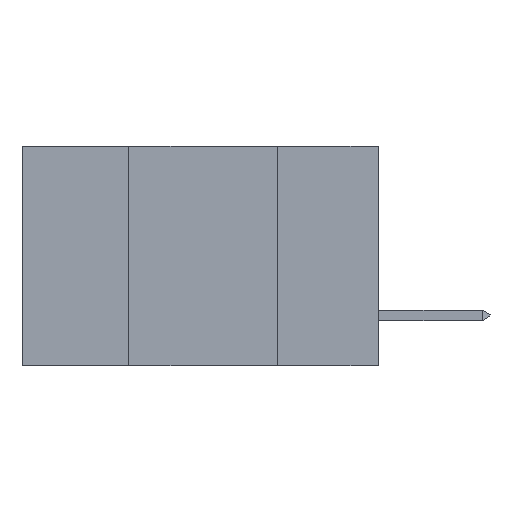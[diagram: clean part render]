
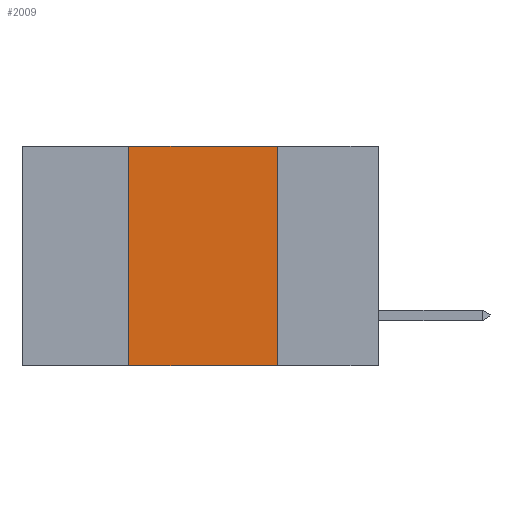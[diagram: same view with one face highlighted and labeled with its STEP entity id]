
A CAD part, left-side view. The second image highlights one B-rep face of the part: STEP entity #2009.
In plain terms, the highlighted planar face has unit normal (-1, 0, 0).
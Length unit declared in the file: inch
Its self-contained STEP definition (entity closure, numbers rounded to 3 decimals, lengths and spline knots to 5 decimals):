
#83 = DIRECTION ( 'NONE',  ( 0., 0., 1. ) ) ;
#159 = LINE ( 'NONE', #3743, #3508 ) ;
#355 = DIRECTION ( 'NONE',  ( 0., -1., 0. ) ) ;
#533 = LINE ( 'NONE', #5887, #10031 ) ;
#777 = EDGE_CURVE ( 'NONE', #8328, #2343, #10930, .T. ) ;
#1561 = VECTOR ( 'NONE', #83, 39.37008 ) ;
#1999 = DIRECTION ( 'NONE',  ( 0., 0., -1. ) ) ;
#2009 = ADVANCED_FACE ( 'NONE', ( #6930 ), #6869, .F. ) ;
#2343 = VERTEX_POINT ( 'NONE', #5089 ) ;
#2747 = CARTESIAN_POINT ( 'NONE',  ( 0., 0.42, 0. ) ) ;
#2966 = ORIENTED_EDGE ( 'NONE', *, *, #777, .T. ) ;
#3103 = EDGE_CURVE ( 'NONE', #8328, #8028, #4557, .T. ) ;
#3508 = VECTOR ( 'NONE', #1999, 39.37008 ) ;
#3743 = CARTESIAN_POINT ( 'NONE',  ( 0., 0.17, -0.37 ) ) ;
#4557 = LINE ( 'NONE', #5515, #1561 ) ;
#4853 = ORIENTED_EDGE ( 'NONE', *, *, #6591, .F. ) ;
#5089 = CARTESIAN_POINT ( 'NONE',  ( 0., 0.17, -0.37 ) ) ;
#5515 = CARTESIAN_POINT ( 'NONE',  ( 0., 0.42, -0.37 ) ) ;
#5874 = CARTESIAN_POINT ( 'NONE',  ( 0., 0.42, -0.37 ) ) ;
#5887 = CARTESIAN_POINT ( 'NONE',  ( 0., 0.6, 0. ) ) ;
#6591 = EDGE_CURVE ( 'NONE', #11062, #2343, #159, .T. ) ;
#6637 = CARTESIAN_POINT ( 'NONE',  ( 0., 0.6, -0.37 ) ) ;
#6811 = CARTESIAN_POINT ( 'NONE',  ( 0., 0.6, 0. ) ) ;
#6869 = PLANE ( 'NONE',  #8933 ) ;
#6930 = FACE_OUTER_BOUND ( 'NONE', #9913, .T. ) ;
#8028 = VERTEX_POINT ( 'NONE', #2747 ) ;
#8328 = VERTEX_POINT ( 'NONE', #5874 ) ;
#8421 = VECTOR ( 'NONE', #9366, 39.37008 ) ;
#8887 = CARTESIAN_POINT ( 'NONE',  ( 0., 0.17, 0. ) ) ;
#8933 = AXIS2_PLACEMENT_3D ( 'NONE', #6811, #10474, #10421 ) ;
#9299 = ORIENTED_EDGE ( 'NONE', *, *, #3103, .F. ) ;
#9366 = DIRECTION ( 'NONE',  ( 0., -1., 0. ) ) ;
#9913 = EDGE_LOOP ( 'NONE', ( #4853, #11368, #9299, #2966 ) ) ;
#10031 = VECTOR ( 'NONE', #355, 39.37008 ) ;
#10075 = EDGE_CURVE ( 'NONE', #8028, #11062, #533, .T. ) ;
#10421 = DIRECTION ( 'NONE',  ( 0., 0., -1. ) ) ;
#10474 = DIRECTION ( 'NONE',  ( 1., 0., 0. ) ) ;
#10930 = LINE ( 'NONE', #6637, #8421 ) ;
#11062 = VERTEX_POINT ( 'NONE', #8887 ) ;
#11368 = ORIENTED_EDGE ( 'NONE', *, *, #10075, .F. ) ;
